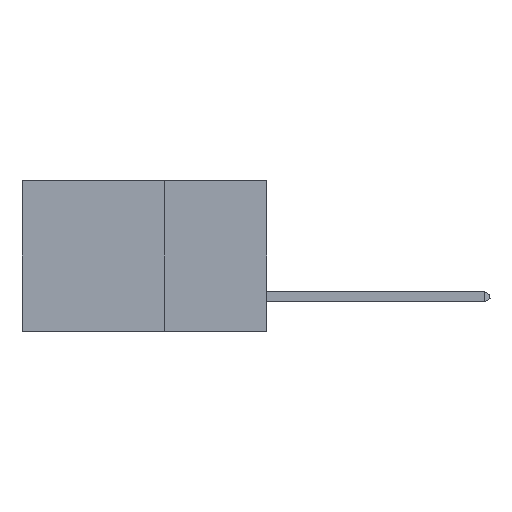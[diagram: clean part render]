
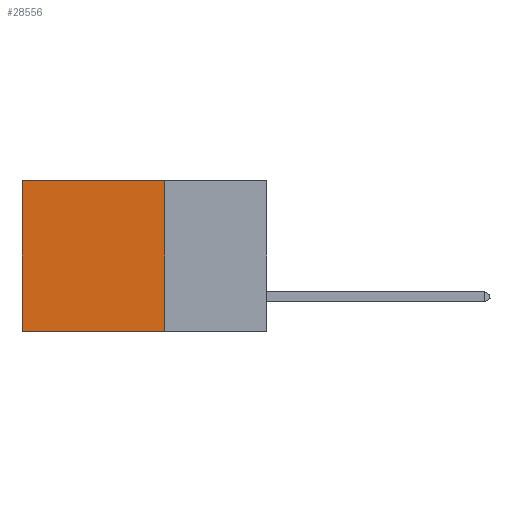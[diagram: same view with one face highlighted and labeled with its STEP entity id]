
A CAD part, left-side view. The second image highlights one B-rep face of the part: STEP entity #28556.
In plain terms, the highlighted planar face has unit normal (-1, 0, 0).
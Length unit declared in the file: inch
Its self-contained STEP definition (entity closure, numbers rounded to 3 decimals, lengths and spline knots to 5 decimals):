
#1818 = DIRECTION ( 'NONE',  ( 0., 0., -1. ) ) ;
#1905 = EDGE_CURVE ( 'NONE', #7796, #21832, #6028, .T. ) ;
#4001 = CARTESIAN_POINT ( 'NONE',  ( 0.2875, 0.25, 0. ) ) ;
#5105 = VECTOR ( 'NONE', #9518, 39.37008 ) ;
#5697 = DIRECTION ( 'NONE',  ( 0., 1., 0. ) ) ;
#5941 = LINE ( 'NONE', #32320, #5105 ) ;
#6028 = LINE ( 'NONE', #32003, #16041 ) ;
#7796 = VERTEX_POINT ( 'NONE', #9936 ) ;
#8149 = FACE_OUTER_BOUND ( 'NONE', #34599, .T. ) ;
#9172 = VECTOR ( 'NONE', #5697, 39.37008 ) ;
#9518 = DIRECTION ( 'NONE',  ( 0., 1., 0. ) ) ;
#9806 = VERTEX_POINT ( 'NONE', #33385 ) ;
#9936 = CARTESIAN_POINT ( 'NONE',  ( 0.2875, 0.25, 0. ) ) ;
#10346 = EDGE_CURVE ( 'NONE', #9806, #22540, #15387, .T. ) ;
#11018 = VECTOR ( 'NONE', #15769, 39.37008 ) ;
#14848 = ORIENTED_EDGE ( 'NONE', *, *, #25144, .T. ) ;
#15387 = LINE ( 'NONE', #24380, #11018 ) ;
#15769 = DIRECTION ( 'NONE',  ( 0., 0., -1. ) ) ;
#16041 = VECTOR ( 'NONE', #1818, 39.37008 ) ;
#17073 = CARTESIAN_POINT ( 'NONE',  ( 0.2875, 0.25, -0.37 ) ) ;
#17483 = ORIENTED_EDGE ( 'NONE', *, *, #1905, .F. ) ;
#17592 = DIRECTION ( 'NONE',  ( 1., 0., 0. ) ) ;
#18520 = AXIS2_PLACEMENT_3D ( 'NONE', #4001, #17592, #31601 ) ;
#19025 = ORIENTED_EDGE ( 'NONE', *, *, #10346, .T. ) ;
#21183 = ORIENTED_EDGE ( 'NONE', *, *, #22803, .F. ) ;
#21832 = VERTEX_POINT ( 'NONE', #26430 ) ;
#22540 = VERTEX_POINT ( 'NONE', #33791 ) ;
#22803 = EDGE_CURVE ( 'NONE', #21832, #22540, #29071, .T. ) ;
#24380 = CARTESIAN_POINT ( 'NONE',  ( 0.2875, 0.6, 0. ) ) ;
#25144 = EDGE_CURVE ( 'NONE', #7796, #9806, #5941, .T. ) ;
#26430 = CARTESIAN_POINT ( 'NONE',  ( 0.2875, 0.25, -0.37 ) ) ;
#28556 = ADVANCED_FACE ( 'NONE', ( #8149 ), #34284, .F. ) ;
#29071 = LINE ( 'NONE', #17073, #9172 ) ;
#31601 = DIRECTION ( 'NONE',  ( 0., 0., -1. ) ) ;
#32003 = CARTESIAN_POINT ( 'NONE',  ( 0.2875, 0.25, 0. ) ) ;
#32320 = CARTESIAN_POINT ( 'NONE',  ( 0.2875, 0.25, 0. ) ) ;
#33385 = CARTESIAN_POINT ( 'NONE',  ( 0.2875, 0.6, 0. ) ) ;
#33791 = CARTESIAN_POINT ( 'NONE',  ( 0.2875, 0.6, -0.37 ) ) ;
#34284 = PLANE ( 'NONE',  #18520 ) ;
#34599 = EDGE_LOOP ( 'NONE', ( #19025, #21183, #17483, #14848 ) ) ;
